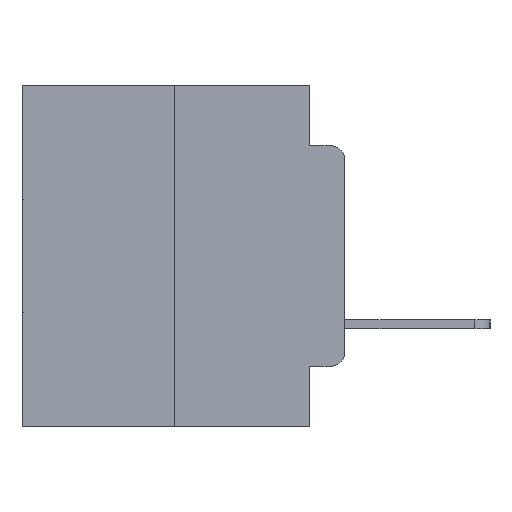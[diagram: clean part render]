
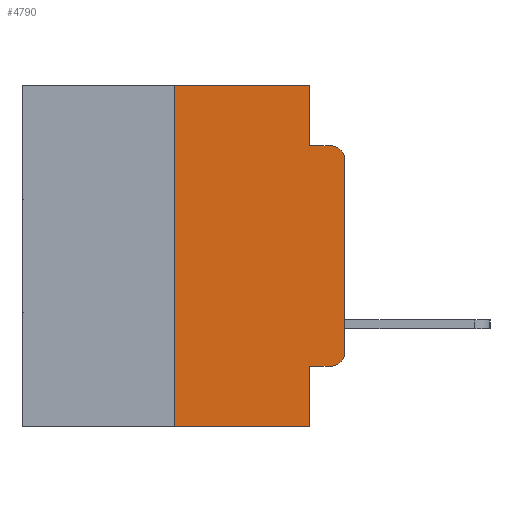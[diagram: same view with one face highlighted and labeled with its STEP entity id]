
A CAD part, left-side view. The second image highlights one B-rep face of the part: STEP entity #4790.
In plain terms, the highlighted planar face has unit normal (-1, 0, 0).
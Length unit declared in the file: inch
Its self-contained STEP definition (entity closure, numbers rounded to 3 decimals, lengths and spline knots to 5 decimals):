
#288 = DIRECTION ( 'NONE',  ( 0., 0., -1. ) ) ;
#1051 = CARTESIAN_POINT ( 'NONE',  ( 0., 0., -0.1085 ) ) ;
#1215 = VECTOR ( 'NONE', #15473, 39.37008 ) ;
#1414 = ORIENTED_EDGE ( 'NONE', *, *, #25067, .T. ) ;
#1584 = CARTESIAN_POINT ( 'NONE',  ( 0., 0.25, -0.5 ) ) ;
#2073 = DIRECTION ( 'NONE',  ( -1., 0., 0. ) ) ;
#2146 = DIRECTION ( 'NONE',  ( -1., 0., 0. ) ) ;
#2397 = DIRECTION ( 'NONE',  ( 1., 0., 0. ) ) ;
#2488 = VECTOR ( 'NONE', #22645, 39.37008 ) ;
#2765 = DIRECTION ( 'NONE',  ( 0., 0., 1. ) ) ;
#3846 = EDGE_CURVE ( 'NONE', #4726, #10234, #19992, .T. ) ;
#4726 = VERTEX_POINT ( 'NONE', #21348 ) ;
#4790 = ADVANCED_FACE ( 'NONE', ( #20723 ), #15299, .F. ) ;
#4904 = CIRCLE ( 'NONE', #16601, 0.02 ) ;
#5073 = LINE ( 'NONE', #7148, #10133 ) ;
#5319 = EDGE_CURVE ( 'NONE', #4726, #7398, #18145, .T. ) ;
#5520 = ORIENTED_EDGE ( 'NONE', *, *, #21265, .T. ) ;
#5930 = LINE ( 'NONE', #20136, #22082 ) ;
#6767 = EDGE_CURVE ( 'NONE', #14775, #15423, #5073, .T. ) ;
#7148 = CARTESIAN_POINT ( 'NONE',  ( 0., 0.25, 0. ) ) ;
#7398 = VERTEX_POINT ( 'NONE', #21955 ) ;
#7538 = ORIENTED_EDGE ( 'NONE', *, *, #21428, .T. ) ;
#8159 = EDGE_LOOP ( 'NONE', ( #1414, #12909, #24607, #14924, #25893, #21718, #5520, #16897, #23651, #7538 ) ) ;
#9388 = CARTESIAN_POINT ( 'NONE',  ( 0., 0.02, -0.4115 ) ) ;
#10133 = VECTOR ( 'NONE', #2765, 39.37008 ) ;
#10234 = VERTEX_POINT ( 'NONE', #9388 ) ;
#10668 = LINE ( 'NONE', #18137, #25994 ) ;
#12536 = VECTOR ( 'NONE', #288, 39.37008 ) ;
#12714 = AXIS2_PLACEMENT_3D ( 'NONE', #15053, #2146, #17166 ) ;
#12729 = LINE ( 'NONE', #13359, #1215 ) ;
#12909 = ORIENTED_EDGE ( 'NONE', *, *, #20922, .T. ) ;
#13170 = CARTESIAN_POINT ( 'NONE',  ( 0., 0.473, 0. ) ) ;
#13238 = CARTESIAN_POINT ( 'NONE',  ( 0., 0.051, 0. ) ) ;
#13359 = CARTESIAN_POINT ( 'NONE',  ( 0., 0., 0. ) ) ;
#13387 = VERTEX_POINT ( 'NONE', #16280 ) ;
#13804 = VECTOR ( 'NONE', #20889, 39.37008 ) ;
#14775 = VERTEX_POINT ( 'NONE', #1584 ) ;
#14924 = ORIENTED_EDGE ( 'NONE', *, *, #15381, .F. ) ;
#14987 = CARTESIAN_POINT ( 'NONE',  ( 0., 0.02, -0.1085 ) ) ;
#15053 = CARTESIAN_POINT ( 'NONE',  ( 0., 0.02, -0.3915 ) ) ;
#15299 = PLANE ( 'NONE',  #17220 ) ;
#15381 = EDGE_CURVE ( 'NONE', #23817, #17005, #17197, .T. ) ;
#15389 = CARTESIAN_POINT ( 'NONE',  ( 0., 0., -0.3915 ) ) ;
#15423 = VERTEX_POINT ( 'NONE', #25399 ) ;
#15473 = DIRECTION ( 'NONE',  ( 0., 0., 1. ) ) ;
#15608 = CIRCLE ( 'NONE', #12714, 0.02 ) ;
#16280 = CARTESIAN_POINT ( 'NONE',  ( 0., 0.02, -0.0885 ) ) ;
#16541 = VECTOR ( 'NONE', #25225, 39.37008 ) ;
#16601 = AXIS2_PLACEMENT_3D ( 'NONE', #14987, #2073, #17094 ) ;
#16801 = EDGE_CURVE ( 'NONE', #17005, #13387, #10668, .T. ) ;
#16897 = ORIENTED_EDGE ( 'NONE', *, *, #5319, .F. ) ;
#17005 = VERTEX_POINT ( 'NONE', #27011 ) ;
#17094 = DIRECTION ( 'NONE',  ( 0., 0., -1. ) ) ;
#17166 = DIRECTION ( 'NONE',  ( 0., 0., -1. ) ) ;
#17197 = LINE ( 'NONE', #27303, #16541 ) ;
#17220 = AXIS2_PLACEMENT_3D ( 'NONE', #13170, #2397, #17405 ) ;
#17405 = DIRECTION ( 'NONE',  ( 0., 0., -1. ) ) ;
#18137 = CARTESIAN_POINT ( 'NONE',  ( 0., 0.051, -0.0885 ) ) ;
#18145 = LINE ( 'NONE', #13238, #12536 ) ;
#18637 = CARTESIAN_POINT ( 'NONE',  ( 0., 0.473, -0.5 ) ) ;
#18696 = VERTEX_POINT ( 'NONE', #1051 ) ;
#19992 = LINE ( 'NONE', #27103, #13804 ) ;
#20136 = CARTESIAN_POINT ( 'NONE',  ( 0., 0.473, 0. ) ) ;
#20723 = FACE_OUTER_BOUND ( 'NONE', #8159, .T. ) ;
#20792 = LINE ( 'NONE', #18637, #2488 ) ;
#20889 = DIRECTION ( 'NONE',  ( 0., -1., 0. ) ) ;
#20922 = EDGE_CURVE ( 'NONE', #18696, #13387, #4904, .T. ) ;
#21108 = EDGE_CURVE ( 'NONE', #15423, #23817, #5930, .T. ) ;
#21265 = EDGE_CURVE ( 'NONE', #14775, #7398, #20792, .T. ) ;
#21348 = CARTESIAN_POINT ( 'NONE',  ( 0., 0.051, -0.4115 ) ) ;
#21428 = EDGE_CURVE ( 'NONE', #10234, #25039, #15608, .T. ) ;
#21718 = ORIENTED_EDGE ( 'NONE', *, *, #6767, .F. ) ;
#21955 = CARTESIAN_POINT ( 'NONE',  ( 0., 0.051, -0.5 ) ) ;
#22082 = VECTOR ( 'NONE', #22200, 39.37008 ) ;
#22200 = DIRECTION ( 'NONE',  ( 0., -1., 0. ) ) ;
#22237 = DIRECTION ( 'NONE',  ( 0., -1., 0. ) ) ;
#22645 = DIRECTION ( 'NONE',  ( 0., -1., 0. ) ) ;
#23651 = ORIENTED_EDGE ( 'NONE', *, *, #3846, .T. ) ;
#23817 = VERTEX_POINT ( 'NONE', #26972 ) ;
#24607 = ORIENTED_EDGE ( 'NONE', *, *, #16801, .F. ) ;
#25039 = VERTEX_POINT ( 'NONE', #15389 ) ;
#25067 = EDGE_CURVE ( 'NONE', #25039, #18696, #12729, .T. ) ;
#25225 = DIRECTION ( 'NONE',  ( 0., 0., -1. ) ) ;
#25399 = CARTESIAN_POINT ( 'NONE',  ( 0., 0.25, 0. ) ) ;
#25893 = ORIENTED_EDGE ( 'NONE', *, *, #21108, .F. ) ;
#25994 = VECTOR ( 'NONE', #22237, 39.37008 ) ;
#26972 = CARTESIAN_POINT ( 'NONE',  ( 0., 0.051, 0. ) ) ;
#27011 = CARTESIAN_POINT ( 'NONE',  ( 0., 0.051, -0.0885 ) ) ;
#27103 = CARTESIAN_POINT ( 'NONE',  ( 0., 0.051, -0.4115 ) ) ;
#27303 = CARTESIAN_POINT ( 'NONE',  ( 0., 0.051, 0. ) ) ;
